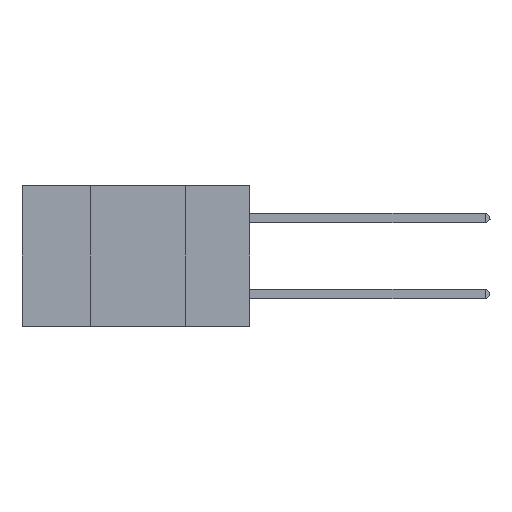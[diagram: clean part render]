
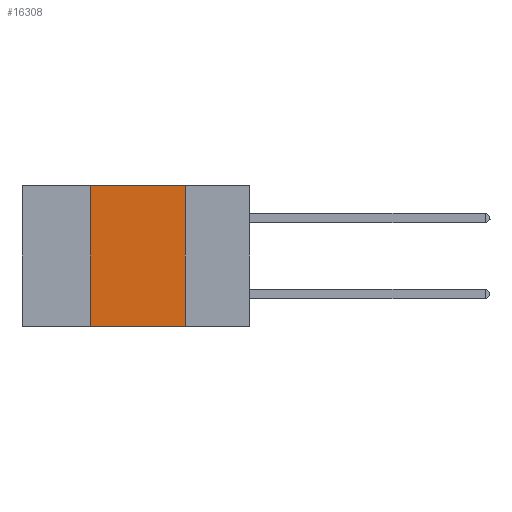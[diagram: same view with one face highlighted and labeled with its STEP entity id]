
A CAD part, left-side view. The second image highlights one B-rep face of the part: STEP entity #16308.
In plain terms, the highlighted planar face has unit normal (-1, 0, 0).
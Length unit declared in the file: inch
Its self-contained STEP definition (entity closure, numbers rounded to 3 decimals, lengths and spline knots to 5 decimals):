
#517 = DIRECTION ( 'NONE',  ( 0., 0., -1. ) ) ;
#1603 = CARTESIAN_POINT ( 'NONE',  ( 0., 0.17, -0.37 ) ) ;
#1646 = EDGE_CURVE ( 'NONE', #8170, #10860, #5541, .T. ) ;
#1855 = VERTEX_POINT ( 'NONE', #9930 ) ;
#2058 = ORIENTED_EDGE ( 'NONE', *, *, #4590, .F. ) ;
#3258 = AXIS2_PLACEMENT_3D ( 'NONE', #3678, #9827, #517 ) ;
#3678 = CARTESIAN_POINT ( 'NONE',  ( 0., 0.6, 0. ) ) ;
#4590 = EDGE_CURVE ( 'NONE', #1855, #9572, #12016, .T. ) ;
#5541 = LINE ( 'NONE', #12757, #13470 ) ;
#6233 = VECTOR ( 'NONE', #7760, 39.37008 ) ;
#6410 = DIRECTION ( 'NONE',  ( 0., 0., -1. ) ) ;
#6542 = CARTESIAN_POINT ( 'NONE',  ( 0., 0.17, 0. ) ) ;
#7255 = EDGE_CURVE ( 'NONE', #10860, #1855, #7708, .T. ) ;
#7615 = VECTOR ( 'NONE', #6410, 39.37008 ) ;
#7708 = LINE ( 'NONE', #10991, #11637 ) ;
#7760 = DIRECTION ( 'NONE',  ( 0., -1., 0. ) ) ;
#8050 = DIRECTION ( 'NONE',  ( 0., -1., 0. ) ) ;
#8170 = VERTEX_POINT ( 'NONE', #8480 ) ;
#8480 = CARTESIAN_POINT ( 'NONE',  ( 0., 0.42, -0.37 ) ) ;
#9448 = EDGE_LOOP ( 'NONE', ( #2058, #14111, #17971, #18417 ) ) ;
#9572 = VERTEX_POINT ( 'NONE', #1603 ) ;
#9827 = DIRECTION ( 'NONE',  ( 1., 0., 0. ) ) ;
#9930 = CARTESIAN_POINT ( 'NONE',  ( 0., 0.17, 0. ) ) ;
#10860 = VERTEX_POINT ( 'NONE', #15208 ) ;
#10991 = CARTESIAN_POINT ( 'NONE',  ( 0., 0.6, 0. ) ) ;
#11637 = VECTOR ( 'NONE', #8050, 39.37008 ) ;
#12016 = LINE ( 'NONE', #6542, #7615 ) ;
#12757 = CARTESIAN_POINT ( 'NONE',  ( 0., 0.42, 0. ) ) ;
#13470 = VECTOR ( 'NONE', #14495, 39.37008 ) ;
#14111 = ORIENTED_EDGE ( 'NONE', *, *, #7255, .F. ) ;
#14495 = DIRECTION ( 'NONE',  ( 0., 0., 1. ) ) ;
#15208 = CARTESIAN_POINT ( 'NONE',  ( 0., 0.42, 0. ) ) ;
#16206 = FACE_OUTER_BOUND ( 'NONE', #9448, .T. ) ;
#16308 = ADVANCED_FACE ( 'NONE', ( #16206 ), #18509, .F. ) ;
#16523 = CARTESIAN_POINT ( 'NONE',  ( 0., 0.6, -0.37 ) ) ;
#17378 = EDGE_CURVE ( 'NONE', #8170, #9572, #17503, .T. ) ;
#17503 = LINE ( 'NONE', #16523, #6233 ) ;
#17971 = ORIENTED_EDGE ( 'NONE', *, *, #1646, .F. ) ;
#18417 = ORIENTED_EDGE ( 'NONE', *, *, #17378, .T. ) ;
#18509 = PLANE ( 'NONE',  #3258 ) ;
